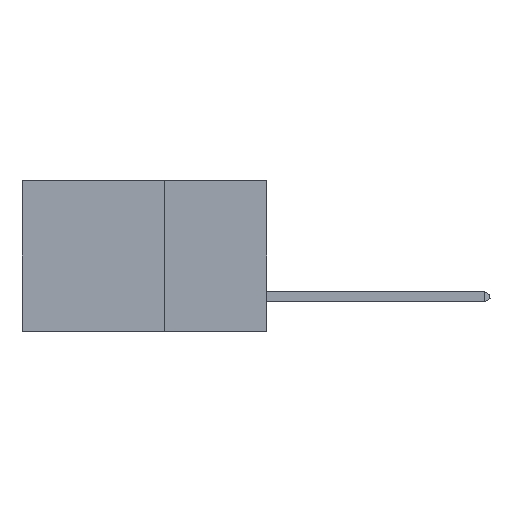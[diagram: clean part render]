
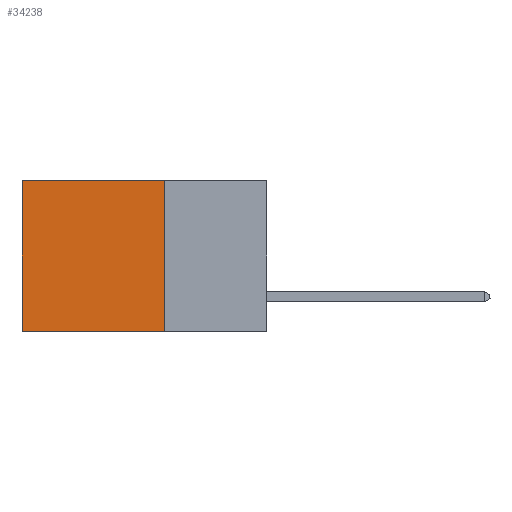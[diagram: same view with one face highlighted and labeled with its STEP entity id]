
A CAD part, left-side view. The second image highlights one B-rep face of the part: STEP entity #34238.
In plain terms, the highlighted planar face has unit normal (-1, 0, 0).
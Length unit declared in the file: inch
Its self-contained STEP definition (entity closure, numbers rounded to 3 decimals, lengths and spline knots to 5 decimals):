
#150 = CARTESIAN_POINT ( 'NONE',  ( 0.2875, 0.25, 0. ) ) ;
#2441 = DIRECTION ( 'NONE',  ( 0., 0., -1. ) ) ;
#2448 = CARTESIAN_POINT ( 'NONE',  ( 0.2875, 0.25, -0.37 ) ) ;
#2586 = CARTESIAN_POINT ( 'NONE',  ( 0.2875, 0.6, 0. ) ) ;
#3747 = DIRECTION ( 'NONE',  ( 0., 0., -1. ) ) ;
#5831 = EDGE_LOOP ( 'NONE', ( #6311, #33855, #36889, #27721 ) ) ;
#6009 = LINE ( 'NONE', #30264, #34733 ) ;
#6311 = ORIENTED_EDGE ( 'NONE', *, *, #34073, .T. ) ;
#6415 = AXIS2_PLACEMENT_3D ( 'NONE', #150, #30511, #21870 ) ;
#7877 = LINE ( 'NONE', #21726, #20909 ) ;
#8892 = EDGE_CURVE ( 'NONE', #15303, #24725, #16703, .T. ) ;
#8974 = DIRECTION ( 'NONE',  ( 0., 1., 0. ) ) ;
#11191 = CARTESIAN_POINT ( 'NONE',  ( 0.2875, 0.6, -0.37 ) ) ;
#15268 = VECTOR ( 'NONE', #3747, 39.37008 ) ;
#15303 = VERTEX_POINT ( 'NONE', #34555 ) ;
#16703 = LINE ( 'NONE', #37342, #15268 ) ;
#18529 = PLANE ( 'NONE',  #6415 ) ;
#20439 = EDGE_CURVE ( 'NONE', #24725, #33902, #32468, .T. ) ;
#20909 = VECTOR ( 'NONE', #8974, 39.37008 ) ;
#21726 = CARTESIAN_POINT ( 'NONE',  ( 0.2875, 0.25, 0. ) ) ;
#21870 = DIRECTION ( 'NONE',  ( 0., 0., -1. ) ) ;
#23002 = EDGE_CURVE ( 'NONE', #15303, #23520, #7877, .T. ) ;
#23520 = VERTEX_POINT ( 'NONE', #2586 ) ;
#24725 = VERTEX_POINT ( 'NONE', #31994 ) ;
#26520 = DIRECTION ( 'NONE',  ( 0., 1., 0. ) ) ;
#27721 = ORIENTED_EDGE ( 'NONE', *, *, #23002, .T. ) ;
#28047 = FACE_OUTER_BOUND ( 'NONE', #5831, .T. ) ;
#30264 = CARTESIAN_POINT ( 'NONE',  ( 0.2875, 0.6, 0. ) ) ;
#30511 = DIRECTION ( 'NONE',  ( 1., 0., 0. ) ) ;
#31483 = VECTOR ( 'NONE', #26520, 39.37008 ) ;
#31994 = CARTESIAN_POINT ( 'NONE',  ( 0.2875, 0.25, -0.37 ) ) ;
#32468 = LINE ( 'NONE', #2448, #31483 ) ;
#33855 = ORIENTED_EDGE ( 'NONE', *, *, #20439, .F. ) ;
#33902 = VERTEX_POINT ( 'NONE', #11191 ) ;
#34073 = EDGE_CURVE ( 'NONE', #23520, #33902, #6009, .T. ) ;
#34238 = ADVANCED_FACE ( 'NONE', ( #28047 ), #18529, .F. ) ;
#34555 = CARTESIAN_POINT ( 'NONE',  ( 0.2875, 0.25, 0. ) ) ;
#34733 = VECTOR ( 'NONE', #2441, 39.37008 ) ;
#36889 = ORIENTED_EDGE ( 'NONE', *, *, #8892, .F. ) ;
#37342 = CARTESIAN_POINT ( 'NONE',  ( 0.2875, 0.25, 0. ) ) ;
